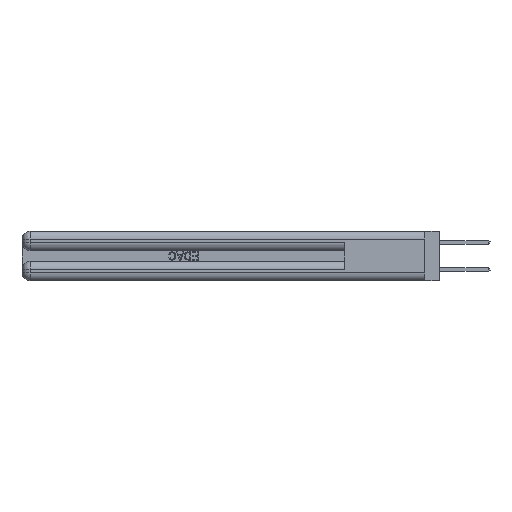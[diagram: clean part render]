
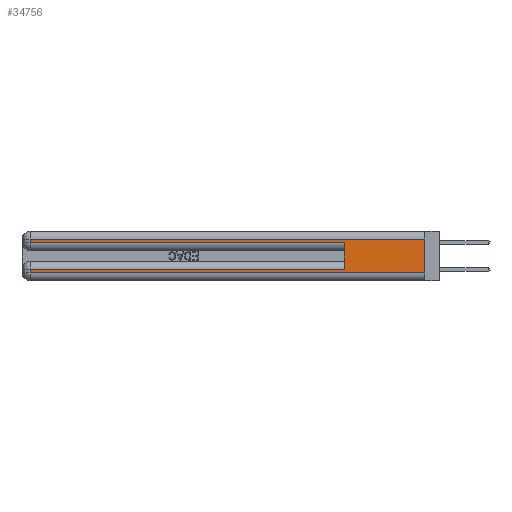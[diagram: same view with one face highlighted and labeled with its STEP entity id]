
A CAD part, left-side view. The second image highlights one B-rep face of the part: STEP entity #34756.
In plain terms, the highlighted planar face has unit normal (-1, 0, 0).
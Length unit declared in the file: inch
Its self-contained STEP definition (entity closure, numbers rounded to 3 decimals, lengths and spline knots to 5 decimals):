
#61 = LINE ( 'NONE', #15125, #36753 ) ;
#1050 = DIRECTION ( 'NONE',  ( 1., 0., 0. ) ) ;
#1444 = DIRECTION ( 'NONE',  ( 0., 0., -1. ) ) ;
#2633 = ORIENTED_EDGE ( 'NONE', *, *, #20674, .T. ) ;
#5500 = CARTESIAN_POINT ( 'NONE',  ( 0., 0., 0.31 ) ) ;
#6031 = LINE ( 'NONE', #34500, #8836 ) ;
#7205 = DIRECTION ( 'NONE',  ( 0., -1., 0. ) ) ;
#7612 = VECTOR ( 'NONE', #37692, 39.37008 ) ;
#7722 = CARTESIAN_POINT ( 'NONE',  ( 0., 0., 0.37 ) ) ;
#7787 = CARTESIAN_POINT ( 'NONE',  ( 0., 2.94, 0.31 ) ) ;
#7957 = AXIS2_PLACEMENT_3D ( 'NONE', #13673, #1050, #1444 ) ;
#7963 = ORIENTED_EDGE ( 'NONE', *, *, #38130, .T. ) ;
#8388 = ORIENTED_EDGE ( 'NONE', *, *, #38762, .T. ) ;
#8836 = VECTOR ( 'NONE', #25658, 39.37008 ) ;
#8929 = EDGE_CURVE ( 'NONE', #28227, #33343, #22723, .T. ) ;
#9132 = ORIENTED_EDGE ( 'NONE', *, *, #30628, .T. ) ;
#9936 = CARTESIAN_POINT ( 'NONE',  ( 0., 2.94, 0.06 ) ) ;
#10250 = VERTEX_POINT ( 'NONE', #11221 ) ;
#11221 = CARTESIAN_POINT ( 'NONE',  ( 0., 0.6, 0.085 ) ) ;
#12115 = CARTESIAN_POINT ( 'NONE',  ( 0., 0., 0.31 ) ) ;
#12461 = LINE ( 'NONE', #36155, #25112 ) ;
#13005 = EDGE_LOOP ( 'NONE', ( #31598, #7963, #9132, #13943, #32077, #8388, #2633, #25324 ) ) ;
#13673 = CARTESIAN_POINT ( 'NONE',  ( 0., 0., 0.37 ) ) ;
#13943 = ORIENTED_EDGE ( 'NONE', *, *, #8929, .T. ) ;
#14570 = VERTEX_POINT ( 'NONE', #36685 ) ;
#15125 = CARTESIAN_POINT ( 'NONE',  ( 0., 0., 0.085 ) ) ;
#15140 = CARTESIAN_POINT ( 'NONE',  ( 0., 2.94, 0.285 ) ) ;
#16438 = VERTEX_POINT ( 'NONE', #37231 ) ;
#17740 = VECTOR ( 'NONE', #35988, 39.37008 ) ;
#18222 = FACE_OUTER_BOUND ( 'NONE', #13005, .T. ) ;
#18866 = EDGE_CURVE ( 'NONE', #36510, #16438, #23567, .T. ) ;
#19035 = PLANE ( 'NONE',  #7957 ) ;
#19192 = LINE ( 'NONE', #33598, #32326 ) ;
#19537 = CARTESIAN_POINT ( 'NONE',  ( 0., 0., 0.285 ) ) ;
#20674 = EDGE_CURVE ( 'NONE', #14570, #24050, #6031, .T. ) ;
#21804 = VECTOR ( 'NONE', #7205, 39.37008 ) ;
#21884 = DIRECTION ( 'NONE',  ( 0., 0., 1. ) ) ;
#22723 = LINE ( 'NONE', #19537, #21804 ) ;
#23567 = LINE ( 'NONE', #7722, #7612 ) ;
#23792 = DIRECTION ( 'NONE',  ( 0., 1., 0. ) ) ;
#23844 = DIRECTION ( 'NONE',  ( 0., 1., 0. ) ) ;
#24050 = VERTEX_POINT ( 'NONE', #9936 ) ;
#25055 = CARTESIAN_POINT ( 'NONE',  ( 0., 0.6, 0.285 ) ) ;
#25112 = VECTOR ( 'NONE', #27290, 39.37008 ) ;
#25324 = ORIENTED_EDGE ( 'NONE', *, *, #35142, .T. ) ;
#25658 = DIRECTION ( 'NONE',  ( 0., 0., -1. ) ) ;
#25685 = LINE ( 'NONE', #36489, #17740 ) ;
#27290 = DIRECTION ( 'NONE',  ( 0., 0., -1. ) ) ;
#28227 = VERTEX_POINT ( 'NONE', #15140 ) ;
#30628 = EDGE_CURVE ( 'NONE', #34407, #28227, #12461, .T. ) ;
#31598 = ORIENTED_EDGE ( 'NONE', *, *, #18866, .F. ) ;
#32077 = ORIENTED_EDGE ( 'NONE', *, *, #33915, .F. ) ;
#32326 = VECTOR ( 'NONE', #21884, 39.37008 ) ;
#33343 = VERTEX_POINT ( 'NONE', #25055 ) ;
#33598 = CARTESIAN_POINT ( 'NONE',  ( 0., 0.6, 0.145 ) ) ;
#33915 = EDGE_CURVE ( 'NONE', #10250, #33343, #19192, .T. ) ;
#34407 = VERTEX_POINT ( 'NONE', #7787 ) ;
#34436 = LINE ( 'NONE', #5500, #37293 ) ;
#34500 = CARTESIAN_POINT ( 'NONE',  ( 0., 2.94, 0.37 ) ) ;
#34756 = ADVANCED_FACE ( 'NONE', ( #18222 ), #19035, .F. ) ;
#35142 = EDGE_CURVE ( 'NONE', #24050, #16438, #25685, .T. ) ;
#35988 = DIRECTION ( 'NONE',  ( 0., -1., 0. ) ) ;
#36155 = CARTESIAN_POINT ( 'NONE',  ( 0., 2.94, 0.37 ) ) ;
#36489 = CARTESIAN_POINT ( 'NONE',  ( 0., 0., 0.06 ) ) ;
#36510 = VERTEX_POINT ( 'NONE', #12115 ) ;
#36685 = CARTESIAN_POINT ( 'NONE',  ( 0., 2.94, 0.085 ) ) ;
#36753 = VECTOR ( 'NONE', #23792, 39.37008 ) ;
#37231 = CARTESIAN_POINT ( 'NONE',  ( 0., 0., 0.06 ) ) ;
#37293 = VECTOR ( 'NONE', #23844, 39.37008 ) ;
#37692 = DIRECTION ( 'NONE',  ( 0., 0., -1. ) ) ;
#38130 = EDGE_CURVE ( 'NONE', #36510, #34407, #34436, .T. ) ;
#38762 = EDGE_CURVE ( 'NONE', #10250, #14570, #61, .T. ) ;
